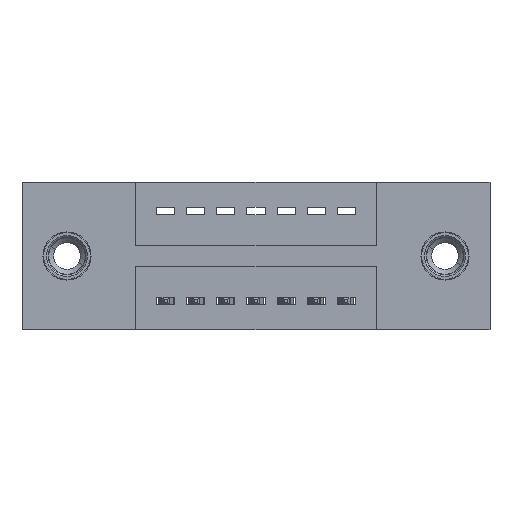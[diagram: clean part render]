
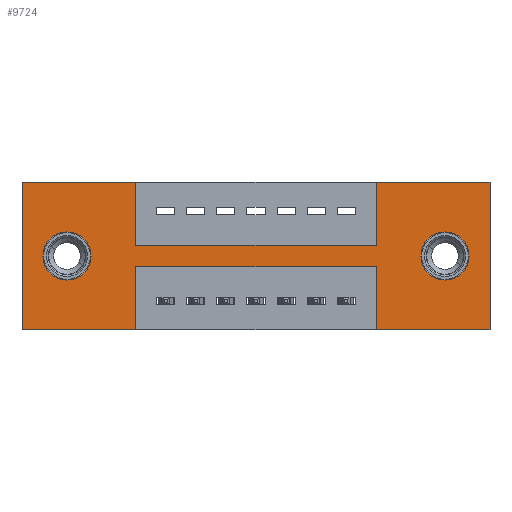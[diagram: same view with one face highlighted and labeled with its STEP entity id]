
A CAD part, front view. The second image highlights one B-rep face of the part: STEP entity #9724.
In plain terms, the highlighted planar face has unit normal (0, -1, 0).
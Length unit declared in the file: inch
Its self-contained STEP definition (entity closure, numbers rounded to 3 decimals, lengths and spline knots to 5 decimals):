
#171 = EDGE_LOOP ( 'NONE', ( #5271, #7468 ) ) ;
#200 = VECTOR ( 'NONE', #731, 39.37008 ) ;
#211 = EDGE_LOOP ( 'NONE', ( #4618, #4399 ) ) ;
#220 = DIRECTION ( 'NONE',  ( 0., 1., 0. ) ) ;
#233 = EDGE_CURVE ( 'NONE', #9960, #4170, #7395, .T. ) ;
#390 = CARTESIAN_POINT ( 'NONE',  ( 0., 0., -0.49 ) ) ;
#472 = EDGE_CURVE ( 'NONE', #1626, #2549, #8937, .T. ) ;
#499 = CARTESIAN_POINT ( 'NONE',  ( 0., 0., -0.49 ) ) ;
#731 = DIRECTION ( 'NONE',  ( -1., 0., 0. ) ) ;
#972 = VECTOR ( 'NONE', #8256, 39.37008 ) ;
#1029 = FACE_BOUND ( 'NONE', #171, .T. ) ;
#1204 = EDGE_CURVE ( 'NONE', #2549, #5266, #8104, .T. ) ;
#1215 = AXIS2_PLACEMENT_3D ( 'NONE', #8754, #220, #4057 ) ;
#1358 = DIRECTION ( 'NONE',  ( 0., 0., 1. ) ) ;
#1439 = DIRECTION ( 'NONE',  ( 0., 1., 0. ) ) ;
#1509 = EDGE_LOOP ( 'NONE', ( #9632, #4086, #9755, #4741, #9880, #4041, #2727, #4386, #5708, #2757, #3845, #7124 ) ) ;
#1551 = DIRECTION ( 'NONE',  ( 0., 0., -1. ) ) ;
#1568 = CARTESIAN_POINT ( 'NONE',  ( 1.1775, 0., -0.21 ) ) ;
#1626 = VERTEX_POINT ( 'NONE', #7771 ) ;
#1702 = CARTESIAN_POINT ( 'NONE',  ( 0.3775, 0., -0.21 ) ) ;
#1741 = FACE_OUTER_BOUND ( 'NONE', #1509, .T. ) ;
#1815 = CIRCLE ( 'NONE', #2954, 0.08 ) ;
#1855 = FACE_BOUND ( 'NONE', #211, .T. ) ;
#1894 = LINE ( 'NONE', #9049, #200 ) ;
#1941 = CARTESIAN_POINT ( 'NONE',  ( 0.3775, 0., -0.49 ) ) ;
#2014 = EDGE_CURVE ( 'NONE', #5185, #4299, #8784, .T. ) ;
#2059 = CIRCLE ( 'NONE', #1215, 0.08 ) ;
#2088 = CARTESIAN_POINT ( 'NONE',  ( 1.555, 0., 0. ) ) ;
#2279 = VERTEX_POINT ( 'NONE', #8220 ) ;
#2286 = AXIS2_PLACEMENT_3D ( 'NONE', #8174, #8790, #6656 ) ;
#2316 = DIRECTION ( 'NONE',  ( 0., 0., 1. ) ) ;
#2540 = DIRECTION ( 'NONE',  ( 0., 0., 1. ) ) ;
#2549 = VERTEX_POINT ( 'NONE', #7808 ) ;
#2727 = ORIENTED_EDGE ( 'NONE', *, *, #1204, .F. ) ;
#2754 = DIRECTION ( 'NONE',  ( 0., 0., -1. ) ) ;
#2757 = ORIENTED_EDGE ( 'NONE', *, *, #8488, .F. ) ;
#2821 = VECTOR ( 'NONE', #7221, 39.37008 ) ;
#2954 = AXIS2_PLACEMENT_3D ( 'NONE', #9446, #9516, #7970 ) ;
#3025 = CARTESIAN_POINT ( 'NONE',  ( 0., 0., 0. ) ) ;
#3044 = LINE ( 'NONE', #7844, #6109 ) ;
#3162 = VECTOR ( 'NONE', #3951, 39.37008 ) ;
#3199 = CARTESIAN_POINT ( 'NONE',  ( 1.1775, 0., 0. ) ) ;
#3257 = EDGE_CURVE ( 'NONE', #4703, #9960, #5036, .T. ) ;
#3258 = VERTEX_POINT ( 'NONE', #5667 ) ;
#3454 = VECTOR ( 'NONE', #2540, 39.37008 ) ;
#3498 = VERTEX_POINT ( 'NONE', #4045 ) ;
#3515 = EDGE_CURVE ( 'NONE', #4299, #7108, #8989, .T. ) ;
#3525 = CIRCLE ( 'NONE', #3626, 0.08 ) ;
#3626 = AXIS2_PLACEMENT_3D ( 'NONE', #7660, #1439, #8503 ) ;
#3738 = DIRECTION ( 'NONE',  ( 1., 0., 0. ) ) ;
#3740 = LINE ( 'NONE', #7276, #9405 ) ;
#3845 = ORIENTED_EDGE ( 'NONE', *, *, #4972, .F. ) ;
#3951 = DIRECTION ( 'NONE',  ( 0., 0., -1. ) ) ;
#4041 = ORIENTED_EDGE ( 'NONE', *, *, #7309, .F. ) ;
#4045 = CARTESIAN_POINT ( 'NONE',  ( 0.1495, 0., -0.325 ) ) ;
#4057 = DIRECTION ( 'NONE',  ( 0., 0., -1. ) ) ;
#4086 = ORIENTED_EDGE ( 'NONE', *, *, #7639, .F. ) ;
#4160 = DIRECTION ( 'NONE',  ( 0., 0., 1. ) ) ;
#4170 = VERTEX_POINT ( 'NONE', #7223 ) ;
#4299 = VERTEX_POINT ( 'NONE', #3199 ) ;
#4304 = EDGE_CURVE ( 'NONE', #4170, #5059, #3044, .T. ) ;
#4386 = ORIENTED_EDGE ( 'NONE', *, *, #472, .F. ) ;
#4399 = ORIENTED_EDGE ( 'NONE', *, *, #5033, .T. ) ;
#4618 = ORIENTED_EDGE ( 'NONE', *, *, #7389, .T. ) ;
#4700 = CARTESIAN_POINT ( 'NONE',  ( 1.4055, 0., -0.165 ) ) ;
#4703 = VERTEX_POINT ( 'NONE', #499 ) ;
#4741 = ORIENTED_EDGE ( 'NONE', *, *, #233, .F. ) ;
#4812 = VECTOR ( 'NONE', #2754, 39.37008 ) ;
#4838 = CARTESIAN_POINT ( 'NONE',  ( 0., 0., 0. ) ) ;
#4907 = CARTESIAN_POINT ( 'NONE',  ( 1.4055, 0., -0.325 ) ) ;
#4972 = EDGE_CURVE ( 'NONE', #7108, #2279, #7311, .T. ) ;
#5033 = EDGE_CURVE ( 'NONE', #3498, #8664, #1815, .T. ) ;
#5036 = LINE ( 'NONE', #9385, #3454 ) ;
#5059 = VERTEX_POINT ( 'NONE', #1702 ) ;
#5082 = EDGE_CURVE ( 'NONE', #7943, #9221, #2059, .T. ) ;
#5185 = VERTEX_POINT ( 'NONE', #7303 ) ;
#5266 = VERTEX_POINT ( 'NONE', #1941 ) ;
#5271 = ORIENTED_EDGE ( 'NONE', *, *, #5614, .T. ) ;
#5333 = LINE ( 'NONE', #8112, #9171 ) ;
#5437 = VECTOR ( 'NONE', #3738, 39.37008 ) ;
#5614 = EDGE_CURVE ( 'NONE', #9221, #7943, #3525, .T. ) ;
#5667 = CARTESIAN_POINT ( 'NONE',  ( 1.1775, 0., -0.49 ) ) ;
#5684 = CARTESIAN_POINT ( 'NONE',  ( 0.3775, 0., -0.28 ) ) ;
#5708 = ORIENTED_EDGE ( 'NONE', *, *, #5888, .F. ) ;
#5888 = EDGE_CURVE ( 'NONE', #3258, #1626, #3740, .T. ) ;
#5936 = CARTESIAN_POINT ( 'NONE',  ( 0.1495, 0., -0.165 ) ) ;
#6109 = VECTOR ( 'NONE', #1551, 39.37008 ) ;
#6351 = DIRECTION ( 'NONE',  ( 1., 0., 0. ) ) ;
#6656 = DIRECTION ( 'NONE',  ( 0., 0., -1. ) ) ;
#7038 = VECTOR ( 'NONE', #9432, 39.37008 ) ;
#7108 = VERTEX_POINT ( 'NONE', #2088 ) ;
#7124 = ORIENTED_EDGE ( 'NONE', *, *, #3515, .F. ) ;
#7221 = DIRECTION ( 'NONE',  ( 1., 0., 0. ) ) ;
#7223 = CARTESIAN_POINT ( 'NONE',  ( 0.3775, 0., 0. ) ) ;
#7276 = CARTESIAN_POINT ( 'NONE',  ( 1.1775, 0., -0.28 ) ) ;
#7303 = CARTESIAN_POINT ( 'NONE',  ( 1.1775, 0., -0.21 ) ) ;
#7309 = EDGE_CURVE ( 'NONE', #5266, #4703, #7523, .T. ) ;
#7311 = LINE ( 'NONE', #9200, #3162 ) ;
#7389 = EDGE_CURVE ( 'NONE', #8664, #3498, #8378, .T. ) ;
#7395 = LINE ( 'NONE', #3025, #5437 ) ;
#7417 = CARTESIAN_POINT ( 'NONE',  ( 0.3775, 0., -0.28 ) ) ;
#7468 = ORIENTED_EDGE ( 'NONE', *, *, #5082, .T. ) ;
#7523 = LINE ( 'NONE', #390, #972 ) ;
#7639 = EDGE_CURVE ( 'NONE', #5059, #5185, #5333, .T. ) ;
#7660 = CARTESIAN_POINT ( 'NONE',  ( 1.4055, 0., -0.245 ) ) ;
#7771 = CARTESIAN_POINT ( 'NONE',  ( 1.1775, 0., -0.28 ) ) ;
#7808 = CARTESIAN_POINT ( 'NONE',  ( 0.3775, 0., -0.28 ) ) ;
#7844 = CARTESIAN_POINT ( 'NONE',  ( 0.3775, 0., -0.21 ) ) ;
#7943 = VERTEX_POINT ( 'NONE', #4907 ) ;
#7970 = DIRECTION ( 'NONE',  ( 0., 0., 1. ) ) ;
#8104 = LINE ( 'NONE', #7417, #4812 ) ;
#8112 = CARTESIAN_POINT ( 'NONE',  ( 0.3775, 0., -0.21 ) ) ;
#8146 = PLANE ( 'NONE',  #2286 ) ;
#8174 = CARTESIAN_POINT ( 'NONE',  ( 0., 0., -0.49 ) ) ;
#8220 = CARTESIAN_POINT ( 'NONE',  ( 1.555, 0., -0.49 ) ) ;
#8256 = DIRECTION ( 'NONE',  ( -1., 0., 0. ) ) ;
#8284 = CARTESIAN_POINT ( 'NONE',  ( 0.1495, 0., -0.245 ) ) ;
#8378 = CIRCLE ( 'NONE', #8452, 0.08 ) ;
#8452 = AXIS2_PLACEMENT_3D ( 'NONE', #8284, #9778, #1358 ) ;
#8488 = EDGE_CURVE ( 'NONE', #2279, #3258, #1894, .T. ) ;
#8503 = DIRECTION ( 'NONE',  ( 0., 0., -1. ) ) ;
#8664 = VERTEX_POINT ( 'NONE', #5936 ) ;
#8754 = CARTESIAN_POINT ( 'NONE',  ( 1.4055, 0., -0.245 ) ) ;
#8784 = LINE ( 'NONE', #1568, #9836 ) ;
#8790 = DIRECTION ( 'NONE',  ( 0., -1., 0. ) ) ;
#8937 = LINE ( 'NONE', #5684, #7038 ) ;
#8989 = LINE ( 'NONE', #4838, #2821 ) ;
#9049 = CARTESIAN_POINT ( 'NONE',  ( 0., 0., -0.49 ) ) ;
#9089 = CARTESIAN_POINT ( 'NONE',  ( 0., 0., 0. ) ) ;
#9171 = VECTOR ( 'NONE', #6351, 39.37008 ) ;
#9200 = CARTESIAN_POINT ( 'NONE',  ( 1.555, 0., 0. ) ) ;
#9221 = VERTEX_POINT ( 'NONE', #4700 ) ;
#9385 = CARTESIAN_POINT ( 'NONE',  ( 0., 0., 0. ) ) ;
#9405 = VECTOR ( 'NONE', #4160, 39.37008 ) ;
#9432 = DIRECTION ( 'NONE',  ( -1., 0., 0. ) ) ;
#9446 = CARTESIAN_POINT ( 'NONE',  ( 0.1495, 0., -0.245 ) ) ;
#9516 = DIRECTION ( 'NONE',  ( 0., 1., 0. ) ) ;
#9632 = ORIENTED_EDGE ( 'NONE', *, *, #2014, .F. ) ;
#9724 = ADVANCED_FACE ( 'NONE', ( #1029, #1855, #1741 ), #8146, .T. ) ;
#9755 = ORIENTED_EDGE ( 'NONE', *, *, #4304, .F. ) ;
#9778 = DIRECTION ( 'NONE',  ( 0., 1., 0. ) ) ;
#9836 = VECTOR ( 'NONE', #2316, 39.37008 ) ;
#9880 = ORIENTED_EDGE ( 'NONE', *, *, #3257, .F. ) ;
#9960 = VERTEX_POINT ( 'NONE', #9089 ) ;
